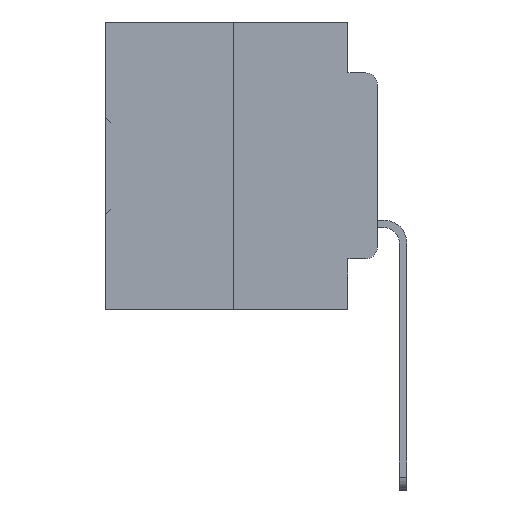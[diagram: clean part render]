
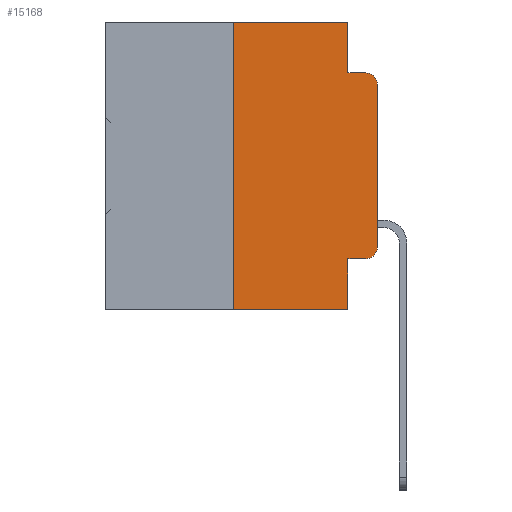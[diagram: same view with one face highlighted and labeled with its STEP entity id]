
A CAD part, left-side view. The second image highlights one B-rep face of the part: STEP entity #15168.
In plain terms, the highlighted planar face has unit normal (-1, 0, 0).
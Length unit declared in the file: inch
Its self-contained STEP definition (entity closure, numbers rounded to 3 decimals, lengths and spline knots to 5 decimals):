
#527 = VECTOR ( 'NONE', #29506, 39.37008 ) ;
#725 = EDGE_CURVE ( 'NONE', #31426, #20647, #24819, .T. ) ;
#779 = VECTOR ( 'NONE', #35296, 39.37008 ) ;
#1729 = VERTEX_POINT ( 'NONE', #4349 ) ;
#2458 = VECTOR ( 'NONE', #2987, 39.37008 ) ;
#2717 = VERTEX_POINT ( 'NONE', #17205 ) ;
#2874 = ORIENTED_EDGE ( 'NONE', *, *, #21194, .T. ) ;
#2876 = DIRECTION ( 'NONE',  ( 1., 0., 0. ) ) ;
#2987 = DIRECTION ( 'NONE',  ( 0., 0., -1. ) ) ;
#3364 = DIRECTION ( 'NONE',  ( -1., 0., 0. ) ) ;
#4349 = CARTESIAN_POINT ( 'NONE',  ( 0., 0.051, -0.4115 ) ) ;
#5729 = AXIS2_PLACEMENT_3D ( 'NONE', #11688, #2876, #23420 ) ;
#6252 = VERTEX_POINT ( 'NONE', #17893 ) ;
#6745 = ORIENTED_EDGE ( 'NONE', *, *, #20162, .T. ) ;
#6948 = CARTESIAN_POINT ( 'NONE',  ( 0., 0.02, -0.3915 ) ) ;
#7020 = EDGE_CURVE ( 'NONE', #10457, #6252, #27867, .T. ) ;
#7469 = VECTOR ( 'NONE', #31767, 39.37008 ) ;
#7578 = LINE ( 'NONE', #20602, #2458 ) ;
#8161 = EDGE_CURVE ( 'NONE', #10457, #13530, #30791, .T. ) ;
#8347 = ORIENTED_EDGE ( 'NONE', *, *, #14253, .T. ) ;
#8397 = LINE ( 'NONE', #9285, #527 ) ;
#8687 = CARTESIAN_POINT ( 'NONE',  ( 0., 0., -0.1085 ) ) ;
#8894 = DIRECTION ( 'NONE',  ( 0., 0., -1. ) ) ;
#9285 = CARTESIAN_POINT ( 'NONE',  ( 0., 0.051, -0.0885 ) ) ;
#9939 = DIRECTION ( 'NONE',  ( 0., 0., -1. ) ) ;
#10087 = CARTESIAN_POINT ( 'NONE',  ( 0., 0.051, 0. ) ) ;
#10457 = VERTEX_POINT ( 'NONE', #20321 ) ;
#10483 = CARTESIAN_POINT ( 'NONE',  ( 0., 0.02, -0.0885 ) ) ;
#11141 = ORIENTED_EDGE ( 'NONE', *, *, #725, .T. ) ;
#11604 = FACE_OUTER_BOUND ( 'NONE', #25223, .T. ) ;
#11688 = CARTESIAN_POINT ( 'NONE',  ( 0., 0.473, 0. ) ) ;
#12051 = DIRECTION ( 'NONE',  ( 0., -1., 0. ) ) ;
#13263 = CARTESIAN_POINT ( 'NONE',  ( 0., 0.051, -0.0885 ) ) ;
#13530 = VERTEX_POINT ( 'NONE', #19911 ) ;
#13571 = CARTESIAN_POINT ( 'NONE',  ( 0., 0.051, -0.4115 ) ) ;
#13779 = CARTESIAN_POINT ( 'NONE',  ( 0., 0., -0.3915 ) ) ;
#14062 = EDGE_CURVE ( 'NONE', #37198, #25472, #36720, .T. ) ;
#14175 = LINE ( 'NONE', #13571, #29498 ) ;
#14253 = EDGE_CURVE ( 'NONE', #2717, #31426, #22217, .T. ) ;
#14787 = ORIENTED_EDGE ( 'NONE', *, *, #27885, .F. ) ;
#15168 = ADVANCED_FACE ( 'NONE', ( #11604 ), #31737, .F. ) ;
#15403 = CARTESIAN_POINT ( 'NONE',  ( 0., 0.25, 0. ) ) ;
#15683 = ORIENTED_EDGE ( 'NONE', *, *, #27934, .F. ) ;
#16075 = EDGE_CURVE ( 'NONE', #25472, #35158, #8397, .T. ) ;
#16907 = ORIENTED_EDGE ( 'NONE', *, *, #8161, .F. ) ;
#17205 = CARTESIAN_POINT ( 'NONE',  ( 0., 0.02, -0.4115 ) ) ;
#17893 = CARTESIAN_POINT ( 'NONE',  ( 0., 0.051, -0.5 ) ) ;
#19911 = CARTESIAN_POINT ( 'NONE',  ( 0., 0.25, 0. ) ) ;
#20162 = EDGE_CURVE ( 'NONE', #1729, #2717, #14175, .T. ) ;
#20213 = VECTOR ( 'NONE', #22304, 39.37008 ) ;
#20321 = CARTESIAN_POINT ( 'NONE',  ( 0., 0.25, -0.5 ) ) ;
#20602 = CARTESIAN_POINT ( 'NONE',  ( 0., 0.051, 0. ) ) ;
#20647 = VERTEX_POINT ( 'NONE', #8687 ) ;
#20983 = CARTESIAN_POINT ( 'NONE',  ( 0., 0.02, -0.1085 ) ) ;
#21194 = EDGE_CURVE ( 'NONE', #20647, #35158, #29002, .T. ) ;
#21780 = VECTOR ( 'NONE', #8894, 39.37008 ) ;
#22217 = CIRCLE ( 'NONE', #33820, 0.02 ) ;
#22304 = DIRECTION ( 'NONE',  ( 0., -1., 0. ) ) ;
#23420 = DIRECTION ( 'NONE',  ( 0., 0., -1. ) ) ;
#23654 = CARTESIAN_POINT ( 'NONE',  ( 0., 0.473, 0. ) ) ;
#23871 = DIRECTION ( 'NONE',  ( 0., 0., -1. ) ) ;
#24819 = LINE ( 'NONE', #32368, #7469 ) ;
#25223 = EDGE_LOOP ( 'NONE', ( #11141, #2874, #30996, #26166, #15683, #16907, #35922, #14787, #6745, #8347 ) ) ;
#25257 = AXIS2_PLACEMENT_3D ( 'NONE', #20983, #3364, #23871 ) ;
#25472 = VERTEX_POINT ( 'NONE', #13263 ) ;
#26166 = ORIENTED_EDGE ( 'NONE', *, *, #14062, .F. ) ;
#27346 = DIRECTION ( 'NONE',  ( -1., 0., 0. ) ) ;
#27867 = LINE ( 'NONE', #30670, #20213 ) ;
#27885 = EDGE_CURVE ( 'NONE', #1729, #6252, #7578, .T. ) ;
#27934 = EDGE_CURVE ( 'NONE', #13530, #37198, #37172, .T. ) ;
#29002 = CIRCLE ( 'NONE', #25257, 0.02 ) ;
#29498 = VECTOR ( 'NONE', #33575, 39.37008 ) ;
#29506 = DIRECTION ( 'NONE',  ( 0., -1., 0. ) ) ;
#30670 = CARTESIAN_POINT ( 'NONE',  ( 0., 0.473, -0.5 ) ) ;
#30791 = LINE ( 'NONE', #15403, #779 ) ;
#30996 = ORIENTED_EDGE ( 'NONE', *, *, #16075, .F. ) ;
#31426 = VERTEX_POINT ( 'NONE', #13779 ) ;
#31737 = PLANE ( 'NONE',  #5729 ) ;
#31767 = DIRECTION ( 'NONE',  ( 0., 0., 1. ) ) ;
#32368 = CARTESIAN_POINT ( 'NONE',  ( 0., 0., 0. ) ) ;
#33575 = DIRECTION ( 'NONE',  ( 0., -1., 0. ) ) ;
#33820 = AXIS2_PLACEMENT_3D ( 'NONE', #6948, #27346, #9939 ) ;
#34632 = CARTESIAN_POINT ( 'NONE',  ( 0., 0.051, 0. ) ) ;
#35158 = VERTEX_POINT ( 'NONE', #10483 ) ;
#35296 = DIRECTION ( 'NONE',  ( 0., 0., 1. ) ) ;
#35431 = VECTOR ( 'NONE', #12051, 39.37008 ) ;
#35922 = ORIENTED_EDGE ( 'NONE', *, *, #7020, .T. ) ;
#36720 = LINE ( 'NONE', #34632, #21780 ) ;
#37172 = LINE ( 'NONE', #23654, #35431 ) ;
#37198 = VERTEX_POINT ( 'NONE', #10087 ) ;
